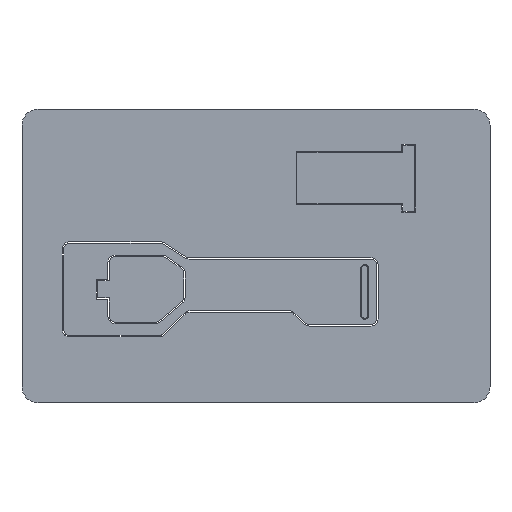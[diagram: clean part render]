
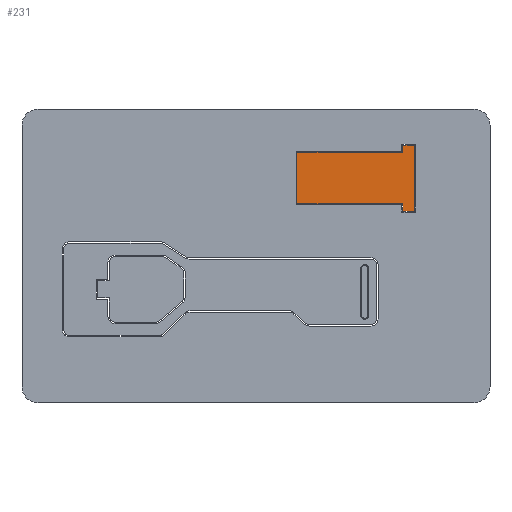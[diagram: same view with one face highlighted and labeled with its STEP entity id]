
A CAD part, front view. The second image highlights one B-rep face of the part: STEP entity #231.
In plain terms, the highlighted planar face has unit normal (0, -1, 0).
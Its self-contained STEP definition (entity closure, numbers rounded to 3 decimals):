
#54 = VECTOR ( 'NONE', #826, 1000. ) ;
#58 = ORIENTED_EDGE ( 'NONE', *, *, #2620, .F. ) ;
#112 = PLANE ( 'NONE',  #3050 ) ;
#145 = VERTEX_POINT ( 'NONE', #580 ) ;
#157 = EDGE_CURVE ( 'NONE', #1598, #2412, #1433, .T. ) ;
#162 = VERTEX_POINT ( 'NONE', #904 ) ;
#231 = ADVANCED_FACE ( 'NONE', ( #682 ), #112, .T. ) ;
#242 = VECTOR ( 'NONE', #2598, 1000. ) ;
#278 = CARTESIAN_POINT ( 'NONE',  ( 64.716, 0., 35.249 ) ) ;
#519 = VECTOR ( 'NONE', #1452, 1000. ) ;
#577 = CARTESIAN_POINT ( 'NONE',  ( 62.536, 0., 24.439 ) ) ;
#580 = CARTESIAN_POINT ( 'NONE',  ( 64.716, 0., 23.079 ) ) ;
#591 = CARTESIAN_POINT ( 'NONE',  ( 62.536, 0., 35.249 ) ) ;
#682 = FACE_OUTER_BOUND ( 'NONE', #1006, .T. ) ;
#781 = ORIENTED_EDGE ( 'NONE', *, *, #157, .F. ) ;
#826 = DIRECTION ( 'NONE',  ( 0., 0., 1. ) ) ;
#904 = CARTESIAN_POINT ( 'NONE',  ( 62.536, 0., 33.889 ) ) ;
#906 = CARTESIAN_POINT ( 'NONE',  ( 43.076, 0., 24.439 ) ) ;
#948 = CARTESIAN_POINT ( 'NONE',  ( 64.716, 0., 35.249 ) ) ;
#1006 = EDGE_LOOP ( 'NONE', ( #3498, #2646, #2688, #781, #2138, #1709, #58, #1548 ) ) ;
#1028 = VERTEX_POINT ( 'NONE', #948 ) ;
#1040 = CARTESIAN_POINT ( 'NONE',  ( 62.536, 0., 24.439 ) ) ;
#1051 = LINE ( 'NONE', #2266, #1367 ) ;
#1106 = EDGE_CURVE ( 'NONE', #3539, #3431, #3250, .T. ) ;
#1212 = VECTOR ( 'NONE', #2407, 1000. ) ;
#1227 = CARTESIAN_POINT ( 'NONE',  ( 62.536, 0., 33.889 ) ) ;
#1236 = EDGE_CURVE ( 'NONE', #2412, #3539, #2375, .T. ) ;
#1279 = CARTESIAN_POINT ( 'NONE',  ( 43.076, 0., 33.889 ) ) ;
#1296 = DIRECTION ( 'NONE',  ( -1., 0., 0. ) ) ;
#1367 = VECTOR ( 'NONE', #1653, 1000. ) ;
#1433 = LINE ( 'NONE', #3787, #242 ) ;
#1452 = DIRECTION ( 'NONE',  ( 0., 0., -1. ) ) ;
#1548 = ORIENTED_EDGE ( 'NONE', *, *, #2103, .F. ) ;
#1598 = VERTEX_POINT ( 'NONE', #3798 ) ;
#1653 = DIRECTION ( 'NONE',  ( 1., 0., 0. ) ) ;
#1709 = ORIENTED_EDGE ( 'NONE', *, *, #2846, .F. ) ;
#1768 = DIRECTION ( 'NONE',  ( 1., 0., 0. ) ) ;
#1834 = CARTESIAN_POINT ( 'NONE',  ( 64.716, 0., 23.079 ) ) ;
#1849 = VERTEX_POINT ( 'NONE', #2587 ) ;
#2058 = LINE ( 'NONE', #591, #3710 ) ;
#2103 = EDGE_CURVE ( 'NONE', #162, #1849, #2964, .T. ) ;
#2110 = DIRECTION ( 'NONE',  ( 0., -1., 0. ) ) ;
#2138 = ORIENTED_EDGE ( 'NONE', *, *, #2309, .F. ) ;
#2260 = VECTOR ( 'NONE', #1296, 1000. ) ;
#2266 = CARTESIAN_POINT ( 'NONE',  ( 43.076, 0., 33.889 ) ) ;
#2309 = EDGE_CURVE ( 'NONE', #145, #1598, #3577, .T. ) ;
#2375 = LINE ( 'NONE', #577, #2814 ) ;
#2407 = DIRECTION ( 'NONE',  ( 0., 0., 1. ) ) ;
#2412 = VERTEX_POINT ( 'NONE', #1040 ) ;
#2587 = CARTESIAN_POINT ( 'NONE',  ( 62.536, 0., 35.249 ) ) ;
#2598 = DIRECTION ( 'NONE',  ( 0., 0., 1. ) ) ;
#2620 = EDGE_CURVE ( 'NONE', #1849, #1028, #2058, .T. ) ;
#2646 = ORIENTED_EDGE ( 'NONE', *, *, #1106, .F. ) ;
#2672 = DIRECTION ( 'NONE',  ( -1., 0., 0. ) ) ;
#2688 = ORIENTED_EDGE ( 'NONE', *, *, #1236, .F. ) ;
#2814 = VECTOR ( 'NONE', #2672, 1000. ) ;
#2846 = EDGE_CURVE ( 'NONE', #1028, #145, #2902, .T. ) ;
#2902 = LINE ( 'NONE', #278, #519 ) ;
#2964 = LINE ( 'NONE', #1227, #1212 ) ;
#3019 = CARTESIAN_POINT ( 'NONE',  ( 75.574, 0., -9.146 ) ) ;
#3050 = AXIS2_PLACEMENT_3D ( 'NONE', #3019, #2110, #3349 ) ;
#3250 = LINE ( 'NONE', #906, #54 ) ;
#3256 = CARTESIAN_POINT ( 'NONE',  ( 43.076, 0., 24.439 ) ) ;
#3349 = DIRECTION ( 'NONE',  ( 0., 0., -1. ) ) ;
#3431 = VERTEX_POINT ( 'NONE', #1279 ) ;
#3498 = ORIENTED_EDGE ( 'NONE', *, *, #3759, .F. ) ;
#3539 = VERTEX_POINT ( 'NONE', #3256 ) ;
#3577 = LINE ( 'NONE', #1834, #2260 ) ;
#3710 = VECTOR ( 'NONE', #1768, 1000. ) ;
#3759 = EDGE_CURVE ( 'NONE', #3431, #162, #1051, .T. ) ;
#3787 = CARTESIAN_POINT ( 'NONE',  ( 62.536, 0., 23.079 ) ) ;
#3798 = CARTESIAN_POINT ( 'NONE',  ( 62.536, 0., 23.079 ) ) ;
